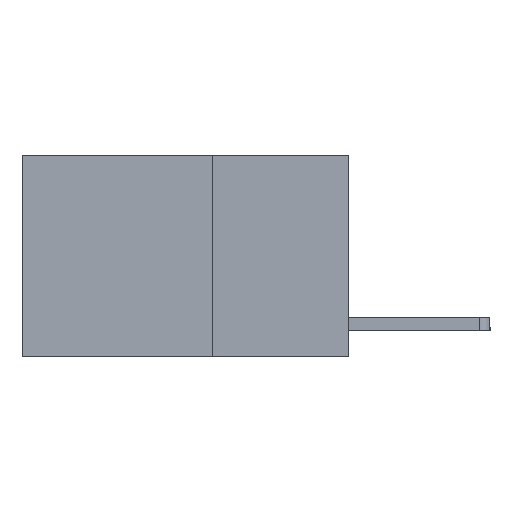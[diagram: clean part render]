
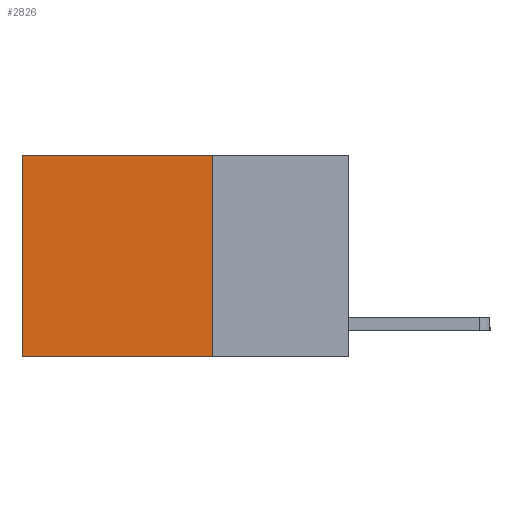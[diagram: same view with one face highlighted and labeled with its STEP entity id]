
A CAD part, left-side view. The second image highlights one B-rep face of the part: STEP entity #2826.
In plain terms, the highlighted planar face has unit normal (-1, 0, 0).
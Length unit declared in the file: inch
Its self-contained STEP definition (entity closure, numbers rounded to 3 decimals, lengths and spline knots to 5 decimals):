
#176 = CARTESIAN_POINT ( 'NONE',  ( 0.2625, 0.25, -0.37 ) ) ;
#213 = VECTOR ( 'NONE', #8719, 39.37008 ) ;
#233 = VERTEX_POINT ( 'NONE', #4654 ) ;
#307 = CARTESIAN_POINT ( 'NONE',  ( 0.2625, 0.25, 0. ) ) ;
#845 = VERTEX_POINT ( 'NONE', #8364 ) ;
#950 = AXIS2_PLACEMENT_3D ( 'NONE', #307, #6960, #10544 ) ;
#1051 = VECTOR ( 'NONE', #3034, 39.37008 ) ;
#1071 = CARTESIAN_POINT ( 'NONE',  ( 0.2625, 0.25, 0. ) ) ;
#1617 = ORIENTED_EDGE ( 'NONE', *, *, #3203, .F. ) ;
#2616 = ORIENTED_EDGE ( 'NONE', *, *, #5010, .F. ) ;
#2826 = ADVANCED_FACE ( 'NONE', ( #6720 ), #11536, .F. ) ;
#3034 = DIRECTION ( 'NONE',  ( 0., 1., 0. ) ) ;
#3064 = VERTEX_POINT ( 'NONE', #6411 ) ;
#3203 = EDGE_CURVE ( 'NONE', #5000, #845, #11647, .T. ) ;
#3222 = EDGE_CURVE ( 'NONE', #3064, #845, #5061, .T. ) ;
#3971 = DIRECTION ( 'NONE',  ( 0., 1., 0. ) ) ;
#4654 = CARTESIAN_POINT ( 'NONE',  ( 0.2625, 0.25, 0. ) ) ;
#4792 = EDGE_LOOP ( 'NONE', ( #8053, #1617, #2616, #10173 ) ) ;
#5000 = VERTEX_POINT ( 'NONE', #5112 ) ;
#5010 = EDGE_CURVE ( 'NONE', #233, #5000, #9701, .T. ) ;
#5061 = LINE ( 'NONE', #6886, #9155 ) ;
#5112 = CARTESIAN_POINT ( 'NONE',  ( 0.2625, 0.25, -0.37 ) ) ;
#6411 = CARTESIAN_POINT ( 'NONE',  ( 0.2625, 0.6, 0. ) ) ;
#6720 = FACE_OUTER_BOUND ( 'NONE', #4792, .T. ) ;
#6886 = CARTESIAN_POINT ( 'NONE',  ( 0.2625, 0.6, 0. ) ) ;
#6960 = DIRECTION ( 'NONE',  ( 1., 0., 0. ) ) ;
#7801 = DIRECTION ( 'NONE',  ( 0., 0., -1. ) ) ;
#8053 = ORIENTED_EDGE ( 'NONE', *, *, #3222, .T. ) ;
#8364 = CARTESIAN_POINT ( 'NONE',  ( 0.2625, 0.6, -0.37 ) ) ;
#8655 = LINE ( 'NONE', #1071, #1051 ) ;
#8719 = DIRECTION ( 'NONE',  ( 0., 0., -1. ) ) ;
#9155 = VECTOR ( 'NONE', #7801, 39.37008 ) ;
#9512 = CARTESIAN_POINT ( 'NONE',  ( 0.2625, 0.25, 0. ) ) ;
#9701 = LINE ( 'NONE', #9512, #213 ) ;
#9750 = VECTOR ( 'NONE', #3971, 39.37008 ) ;
#9856 = EDGE_CURVE ( 'NONE', #233, #3064, #8655, .T. ) ;
#10173 = ORIENTED_EDGE ( 'NONE', *, *, #9856, .T. ) ;
#10544 = DIRECTION ( 'NONE',  ( 0., 0., -1. ) ) ;
#11536 = PLANE ( 'NONE',  #950 ) ;
#11647 = LINE ( 'NONE', #176, #9750 ) ;
